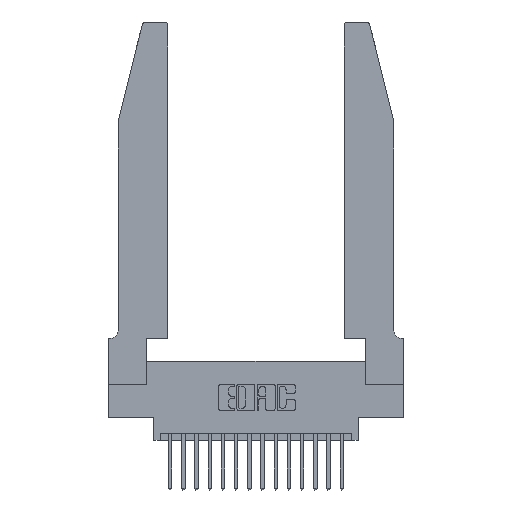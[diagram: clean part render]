
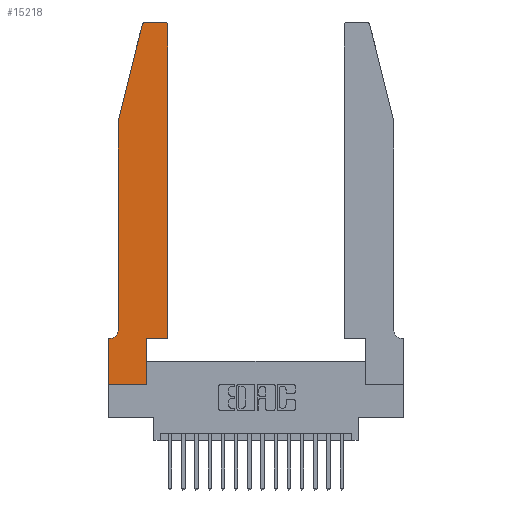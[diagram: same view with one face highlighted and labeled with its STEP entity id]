
A CAD part, top view. The second image highlights one B-rep face of the part: STEP entity #15218.
In plain terms, the highlighted planar face has unit normal (0, 0, 1).
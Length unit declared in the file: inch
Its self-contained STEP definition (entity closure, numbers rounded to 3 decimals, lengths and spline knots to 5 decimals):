
#203 = EDGE_CURVE ( 'NONE', #5531, #11800, #9360, .T. ) ;
#292 = EDGE_CURVE ( 'NONE', #13975, #11924, #10566, .T. ) ;
#933 = CIRCLE ( 'NONE', #9385, 0.07 ) ;
#1650 = LINE ( 'NONE', #5983, #5881 ) ;
#1737 = ORIENTED_EDGE ( 'NONE', *, *, #203, .T. ) ;
#1918 = CARTESIAN_POINT ( 'NONE',  ( 0.4205, 2.75, 0.37 ) ) ;
#2186 = VECTOR ( 'NONE', #3736, 39.37008 ) ;
#2243 = AXIS2_PLACEMENT_3D ( 'NONE', #3915, #2476, #2346 ) ;
#2293 = LINE ( 'NONE', #9396, #2777 ) ;
#2346 = DIRECTION ( 'NONE',  ( 1., 0., 0. ) ) ;
#2358 = EDGE_CURVE ( 'NONE', #19230, #9278, #3400, .T. ) ;
#2476 = DIRECTION ( 'NONE',  ( 0., 0., 1. ) ) ;
#2564 = DIRECTION ( 'NONE',  ( 1., 0., 0. ) ) ;
#2777 = VECTOR ( 'NONE', #14727, 39.37008 ) ;
#3009 = LINE ( 'NONE', #11662, #16574 ) ;
#3400 = LINE ( 'NONE', #14763, #15031 ) ;
#3602 = CARTESIAN_POINT ( 'NONE',  ( 0.2605, 2.75, 0.37 ) ) ;
#3736 = DIRECTION ( 'NONE',  ( -1., 0., 0. ) ) ;
#3903 = DIRECTION ( 'NONE',  ( 0., 0., 1. ) ) ;
#3915 = CARTESIAN_POINT ( 'NONE',  ( 0.4205, 2.72, 0.37 ) ) ;
#4175 = CARTESIAN_POINT ( 'NONE',  ( 0., 0.35, 0.37 ) ) ;
#4282 = ORIENTED_EDGE ( 'NONE', *, *, #6176, .T. ) ;
#4691 = CARTESIAN_POINT ( 'NONE',  ( 0., 0., 0.37 ) ) ;
#5114 = ORIENTED_EDGE ( 'NONE', *, *, #10346, .T. ) ;
#5196 = CARTESIAN_POINT ( 'NONE',  ( 0.0055, 0.42, 0.37 ) ) ;
#5260 = DIRECTION ( 'NONE',  ( -1., 0., 0. ) ) ;
#5367 = DIRECTION ( 'NONE',  ( -1., 0., 0. ) ) ;
#5400 = CIRCLE ( 'NONE', #2243, 0.03 ) ;
#5531 = VERTEX_POINT ( 'NONE', #10493 ) ;
#5756 = PLANE ( 'NONE',  #11369 ) ;
#5793 = EDGE_CURVE ( 'NONE', #6069, #17107, #5400, .T. ) ;
#5881 = VECTOR ( 'NONE', #15097, 39.37008 ) ;
#5983 = CARTESIAN_POINT ( 'NONE',  ( 0.2865, 0.35, 0.37 ) ) ;
#6069 = VERTEX_POINT ( 'NONE', #16329 ) ;
#6176 = EDGE_CURVE ( 'NONE', #11924, #5531, #933, .T. ) ;
#6705 = FACE_OUTER_BOUND ( 'NONE', #10688, .T. ) ;
#6751 = CARTESIAN_POINT ( 'NONE',  ( 0.2865, 0.35, 0.37 ) ) ;
#6899 = EDGE_CURVE ( 'NONE', #11800, #10409, #2293, .T. ) ;
#7167 = CARTESIAN_POINT ( 'NONE',  ( 0.0755, 2., 0.37 ) ) ;
#7281 = EDGE_CURVE ( 'NONE', #9671, #13975, #15584, .T. ) ;
#7306 = AXIS2_PLACEMENT_3D ( 'NONE', #19249, #3903, #16200 ) ;
#7384 = DIRECTION ( 'NONE',  ( 1., 0., 0. ) ) ;
#7626 = DIRECTION ( 'NONE',  ( 0., -1., 0. ) ) ;
#7647 = DIRECTION ( 'NONE',  ( -0.239, -0.971, 0. ) ) ;
#7693 = CARTESIAN_POINT ( 'NONE',  ( 0.0755, 2., 0.37 ) ) ;
#7898 = CARTESIAN_POINT ( 'NONE',  ( 0.25487, 2.72718, 0.37 ) ) ;
#8707 = VERTEX_POINT ( 'NONE', #17654 ) ;
#8775 = CARTESIAN_POINT ( 'NONE',  ( 0.4505, 0.35, 0.37 ) ) ;
#9278 = VERTEX_POINT ( 'NONE', #12451 ) ;
#9358 = LINE ( 'NONE', #3602, #2186 ) ;
#9360 = LINE ( 'NONE', #9940, #19429 ) ;
#9385 = AXIS2_PLACEMENT_3D ( 'NONE', #5196, #15833, #5260 ) ;
#9396 = CARTESIAN_POINT ( 'NONE',  ( 0., 0., 0.37 ) ) ;
#9671 = VERTEX_POINT ( 'NONE', #7898 ) ;
#9940 = CARTESIAN_POINT ( 'NONE',  ( 0.0755, 0.35, 0.37 ) ) ;
#10346 = EDGE_CURVE ( 'NONE', #9278, #6069, #10720, .T. ) ;
#10409 = VERTEX_POINT ( 'NONE', #4691 ) ;
#10426 = ORIENTED_EDGE ( 'NONE', *, *, #292, .T. ) ;
#10493 = CARTESIAN_POINT ( 'NONE',  ( 0.0055, 0.35, 0.37 ) ) ;
#10566 = LINE ( 'NONE', #7693, #15336 ) ;
#10688 = EDGE_LOOP ( 'NONE', ( #19029, #18641, #17023, #10426, #4282, #1737, #11722, #14900, #10962, #14198, #5114, #12341 ) ) ;
#10720 = LINE ( 'NONE', #8775, #18405 ) ;
#10859 = CARTESIAN_POINT ( 'NONE',  ( 0., 0.35, 0.37 ) ) ;
#10962 = ORIENTED_EDGE ( 'NONE', *, *, #17505, .T. ) ;
#11369 = AXIS2_PLACEMENT_3D ( 'NONE', #4175, #17827, #13682 ) ;
#11628 = VERTEX_POINT ( 'NONE', #12140 ) ;
#11662 = CARTESIAN_POINT ( 'NONE',  ( 0., 0., 0.37 ) ) ;
#11722 = ORIENTED_EDGE ( 'NONE', *, *, #6899, .T. ) ;
#11800 = VERTEX_POINT ( 'NONE', #10859 ) ;
#11924 = VERTEX_POINT ( 'NONE', #15782 ) ;
#12140 = CARTESIAN_POINT ( 'NONE',  ( 0.2865, 0., 0.37 ) ) ;
#12239 = CARTESIAN_POINT ( 'NONE',  ( 0.0755, 2., 0.37 ) ) ;
#12341 = ORIENTED_EDGE ( 'NONE', *, *, #5793, .T. ) ;
#12451 = CARTESIAN_POINT ( 'NONE',  ( 0.4505, 0.35, 0.37 ) ) ;
#12544 = EDGE_CURVE ( 'NONE', #17107, #8707, #9358, .T. ) ;
#13196 = VECTOR ( 'NONE', #7647, 39.37008 ) ;
#13318 = EDGE_CURVE ( 'NONE', #10409, #11628, #3009, .T. ) ;
#13682 = DIRECTION ( 'NONE',  ( 1., 0., 0. ) ) ;
#13975 = VERTEX_POINT ( 'NONE', #7167 ) ;
#14198 = ORIENTED_EDGE ( 'NONE', *, *, #2358, .T. ) ;
#14727 = DIRECTION ( 'NONE',  ( 0., -1., 0. ) ) ;
#14763 = CARTESIAN_POINT ( 'NONE',  ( 0.4505, 0.35, 0.37 ) ) ;
#14900 = ORIENTED_EDGE ( 'NONE', *, *, #13318, .T. ) ;
#15031 = VECTOR ( 'NONE', #2564, 39.37008 ) ;
#15097 = DIRECTION ( 'NONE',  ( 0., 1., 0. ) ) ;
#15218 = ADVANCED_FACE ( 'NONE', ( #6705 ), #5756, .T. ) ;
#15336 = VECTOR ( 'NONE', #7626, 39.37008 ) ;
#15584 = LINE ( 'NONE', #12239, #13196 ) ;
#15782 = CARTESIAN_POINT ( 'NONE',  ( 0.0755, 0.42, 0.37 ) ) ;
#15833 = DIRECTION ( 'NONE',  ( 0., 0., -1. ) ) ;
#16200 = DIRECTION ( 'NONE',  ( 1., 0., 0. ) ) ;
#16329 = CARTESIAN_POINT ( 'NONE',  ( 0.4505, 2.72, 0.37 ) ) ;
#16392 = DIRECTION ( 'NONE',  ( 0., 1., 0. ) ) ;
#16574 = VECTOR ( 'NONE', #7384, 39.37008 ) ;
#16731 = EDGE_CURVE ( 'NONE', #8707, #9671, #17122, .T. ) ;
#17023 = ORIENTED_EDGE ( 'NONE', *, *, #7281, .T. ) ;
#17107 = VERTEX_POINT ( 'NONE', #1918 ) ;
#17122 = CIRCLE ( 'NONE', #7306, 0.03 ) ;
#17505 = EDGE_CURVE ( 'NONE', #11628, #19230, #1650, .T. ) ;
#17654 = CARTESIAN_POINT ( 'NONE',  ( 0.284, 2.75, 0.37 ) ) ;
#17827 = DIRECTION ( 'NONE',  ( 0., 0., 1. ) ) ;
#18405 = VECTOR ( 'NONE', #16392, 39.37008 ) ;
#18641 = ORIENTED_EDGE ( 'NONE', *, *, #16731, .T. ) ;
#19029 = ORIENTED_EDGE ( 'NONE', *, *, #12544, .T. ) ;
#19230 = VERTEX_POINT ( 'NONE', #6751 ) ;
#19249 = CARTESIAN_POINT ( 'NONE',  ( 0.284, 2.72, 0.37 ) ) ;
#19429 = VECTOR ( 'NONE', #5367, 39.37008 ) ;
